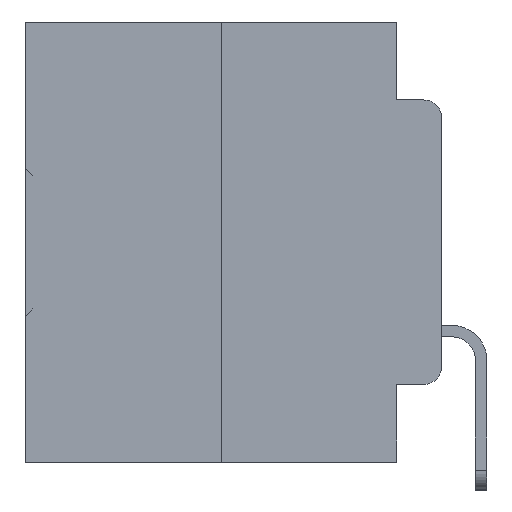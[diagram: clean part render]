
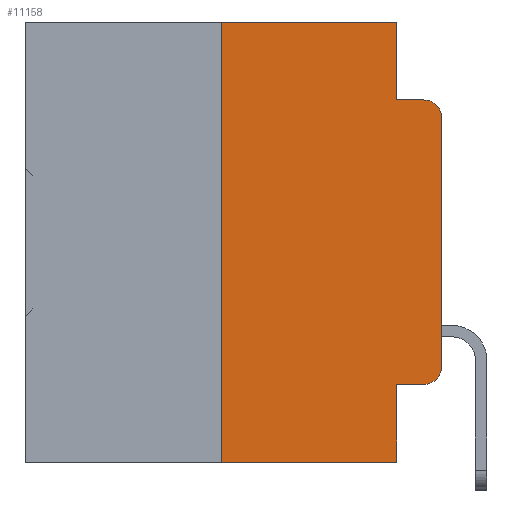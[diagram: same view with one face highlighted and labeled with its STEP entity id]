
A CAD part, left-side view. The second image highlights one B-rep face of the part: STEP entity #11158.
In plain terms, the highlighted planar face has unit normal (-1, 0, 0).
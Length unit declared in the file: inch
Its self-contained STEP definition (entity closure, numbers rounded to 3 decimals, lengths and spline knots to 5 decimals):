
#722 = EDGE_CURVE ( 'NONE', #25413, #30975, #30029, .T. ) ;
#826 = ORIENTED_EDGE ( 'NONE', *, *, #22326, .F. ) ;
#1804 = DIRECTION ( 'NONE',  ( -1., 0., 0. ) ) ;
#2042 = LINE ( 'NONE', #3608, #31745 ) ;
#2183 = ORIENTED_EDGE ( 'NONE', *, *, #722, .T. ) ;
#2378 = ORIENTED_EDGE ( 'NONE', *, *, #28274, .T. ) ;
#2604 = LINE ( 'NONE', #10919, #10726 ) ;
#2691 = ORIENTED_EDGE ( 'NONE', *, *, #5213, .T. ) ;
#3213 = CARTESIAN_POINT ( 'NONE',  ( 0., 0.25, 0. ) ) ;
#3608 = CARTESIAN_POINT ( 'NONE',  ( 0., 0.051, 0. ) ) ;
#4710 = CARTESIAN_POINT ( 'NONE',  ( 0., 0.051, -0.0885 ) ) ;
#5213 = EDGE_CURVE ( 'NONE', #27564, #19473, #15195, .T. ) ;
#5602 = ORIENTED_EDGE ( 'NONE', *, *, #29045, .F. ) ;
#6537 = VERTEX_POINT ( 'NONE', #23309 ) ;
#6682 = DIRECTION ( 'NONE',  ( 0., 0., -1. ) ) ;
#6897 = ORIENTED_EDGE ( 'NONE', *, *, #24668, .T. ) ;
#7541 = ORIENTED_EDGE ( 'NONE', *, *, #7752, .T. ) ;
#7752 = EDGE_CURVE ( 'NONE', #11317, #29316, #34430, .T. ) ;
#7931 = DIRECTION ( 'NONE',  ( 0., 0., 1. ) ) ;
#9750 = ORIENTED_EDGE ( 'NONE', *, *, #22002, .F. ) ;
#9906 = VECTOR ( 'NONE', #22237, 39.37008 ) ;
#10140 = DIRECTION ( 'NONE',  ( 0., 0., -1. ) ) ;
#10726 = VECTOR ( 'NONE', #7931, 39.37008 ) ;
#10919 = CARTESIAN_POINT ( 'NONE',  ( 0., 0., 0. ) ) ;
#11082 = EDGE_CURVE ( 'NONE', #35069, #18987, #2042, .T. ) ;
#11158 = ADVANCED_FACE ( 'NONE', ( #14365 ), #24396, .F. ) ;
#11317 = VERTEX_POINT ( 'NONE', #16825 ) ;
#11509 = VERTEX_POINT ( 'NONE', #26065 ) ;
#11624 = DIRECTION ( 'NONE',  ( 0., -1., 0. ) ) ;
#11639 = LINE ( 'NONE', #20420, #19237 ) ;
#13191 = CARTESIAN_POINT ( 'NONE',  ( 0., 0.25, -0.5 ) ) ;
#13193 = CARTESIAN_POINT ( 'NONE',  ( 0., 0.02, -0.1085 ) ) ;
#13564 = ORIENTED_EDGE ( 'NONE', *, *, #11082, .F. ) ;
#13999 = LINE ( 'NONE', #28461, #20618 ) ;
#14365 = FACE_OUTER_BOUND ( 'NONE', #16570, .T. ) ;
#14390 = AXIS2_PLACEMENT_3D ( 'NONE', #13193, #32673, #16091 ) ;
#14744 = DIRECTION ( 'NONE',  ( 0., 0., -1. ) ) ;
#15195 = LINE ( 'NONE', #15579, #26535 ) ;
#15579 = CARTESIAN_POINT ( 'NONE',  ( 0., 0.473, -0.5 ) ) ;
#15733 = EDGE_CURVE ( 'NONE', #18987, #30975, #22971, .T. ) ;
#16091 = DIRECTION ( 'NONE',  ( 0., 0., -1. ) ) ;
#16262 = ORIENTED_EDGE ( 'NONE', *, *, #15733, .F. ) ;
#16570 = EDGE_LOOP ( 'NONE', ( #2378, #2183, #16262, #13564, #9750, #826, #2691, #5602, #6897, #7541 ) ) ;
#16825 = CARTESIAN_POINT ( 'NONE',  ( 0., 0.02, -0.4115 ) ) ;
#17725 = LINE ( 'NONE', #19412, #9906 ) ;
#18987 = VERTEX_POINT ( 'NONE', #4710 ) ;
#19237 = VECTOR ( 'NONE', #14744, 39.37008 ) ;
#19412 = CARTESIAN_POINT ( 'NONE',  ( 0., 0.473, 0. ) ) ;
#19473 = VERTEX_POINT ( 'NONE', #29732 ) ;
#19579 = CARTESIAN_POINT ( 'NONE',  ( 0., 0.02, -0.3915 ) ) ;
#20360 = CARTESIAN_POINT ( 'NONE',  ( 0., 0., -0.1085 ) ) ;
#20420 = CARTESIAN_POINT ( 'NONE',  ( 0., 0.051, 0. ) ) ;
#20618 = VECTOR ( 'NONE', #11624, 39.37008 ) ;
#21189 = CARTESIAN_POINT ( 'NONE',  ( 0., 0.051, 0. ) ) ;
#22002 = EDGE_CURVE ( 'NONE', #6537, #35069, #17725, .T. ) ;
#22237 = DIRECTION ( 'NONE',  ( 0., -1., 0. ) ) ;
#22326 = EDGE_CURVE ( 'NONE', #27564, #6537, #34913, .T. ) ;
#22377 = DIRECTION ( 'NONE',  ( 0., 0., -1. ) ) ;
#22971 = LINE ( 'NONE', #32541, #28584 ) ;
#23309 = CARTESIAN_POINT ( 'NONE',  ( 0., 0.25, 0. ) ) ;
#24242 = DIRECTION ( 'NONE',  ( 0., -1., 0. ) ) ;
#24396 = PLANE ( 'NONE',  #34470 ) ;
#24668 = EDGE_CURVE ( 'NONE', #11509, #11317, #13999, .T. ) ;
#25413 = VERTEX_POINT ( 'NONE', #20360 ) ;
#26065 = CARTESIAN_POINT ( 'NONE',  ( 0., 0.051, -0.4115 ) ) ;
#26535 = VECTOR ( 'NONE', #26784, 39.37008 ) ;
#26784 = DIRECTION ( 'NONE',  ( 0., -1., 0. ) ) ;
#27169 = DIRECTION ( 'NONE',  ( 1., 0., 0. ) ) ;
#27536 = AXIS2_PLACEMENT_3D ( 'NONE', #19579, #1804, #22377 ) ;
#27564 = VERTEX_POINT ( 'NONE', #13191 ) ;
#28274 = EDGE_CURVE ( 'NONE', #29316, #25413, #2604, .T. ) ;
#28461 = CARTESIAN_POINT ( 'NONE',  ( 0., 0.051, -0.4115 ) ) ;
#28584 = VECTOR ( 'NONE', #24242, 39.37008 ) ;
#29045 = EDGE_CURVE ( 'NONE', #11509, #19473, #11639, .T. ) ;
#29316 = VERTEX_POINT ( 'NONE', #35172 ) ;
#29732 = CARTESIAN_POINT ( 'NONE',  ( 0., 0.051, -0.5 ) ) ;
#30029 = CIRCLE ( 'NONE', #14390, 0.02 ) ;
#30975 = VERTEX_POINT ( 'NONE', #37124 ) ;
#31745 = VECTOR ( 'NONE', #6682, 39.37008 ) ;
#31944 = DIRECTION ( 'NONE',  ( 0., 0., 1. ) ) ;
#32541 = CARTESIAN_POINT ( 'NONE',  ( 0., 0.051, -0.0885 ) ) ;
#32673 = DIRECTION ( 'NONE',  ( -1., 0., 0. ) ) ;
#34430 = CIRCLE ( 'NONE', #27536, 0.02 ) ;
#34470 = AXIS2_PLACEMENT_3D ( 'NONE', #35274, #27169, #10140 ) ;
#34913 = LINE ( 'NONE', #3213, #35768 ) ;
#35069 = VERTEX_POINT ( 'NONE', #21189 ) ;
#35172 = CARTESIAN_POINT ( 'NONE',  ( 0., 0., -0.3915 ) ) ;
#35274 = CARTESIAN_POINT ( 'NONE',  ( 0., 0.473, 0. ) ) ;
#35768 = VECTOR ( 'NONE', #31944, 39.37008 ) ;
#37124 = CARTESIAN_POINT ( 'NONE',  ( 0., 0.02, -0.0885 ) ) ;
